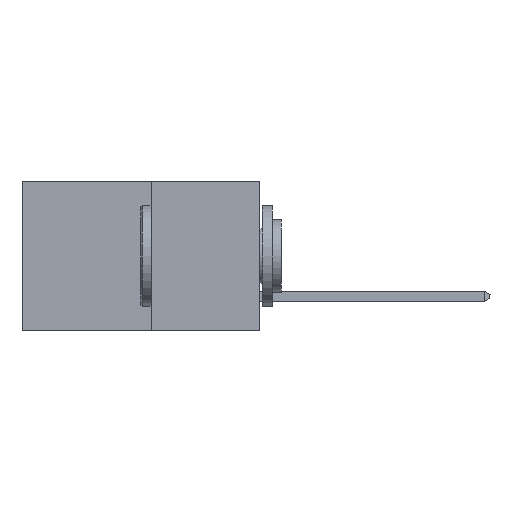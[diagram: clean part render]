
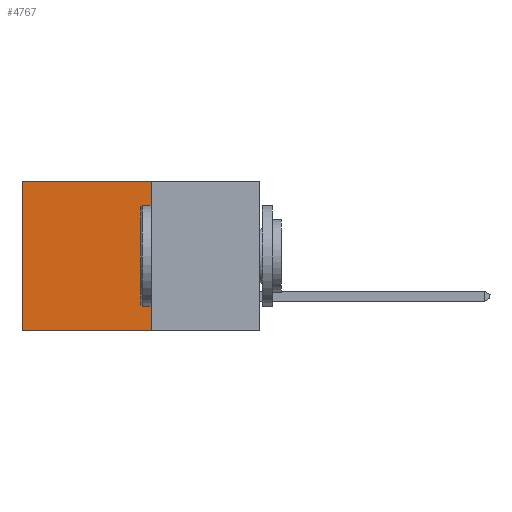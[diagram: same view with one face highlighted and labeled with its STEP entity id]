
A CAD part, left-side view. The second image highlights one B-rep face of the part: STEP entity #4767.
In plain terms, the highlighted planar face has unit normal (-1, 0, 0).
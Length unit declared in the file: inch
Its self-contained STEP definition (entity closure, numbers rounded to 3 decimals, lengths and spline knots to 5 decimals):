
#166 = CARTESIAN_POINT ( 'NONE',  ( 0.277, 0.27, -0.37 ) ) ;
#188 = CARTESIAN_POINT ( 'NONE',  ( 0.277, 0.27, 0. ) ) ;
#253 = FACE_OUTER_BOUND ( 'NONE', #12273, .T. ) ;
#357 = ORIENTED_EDGE ( 'NONE', *, *, #11550, .T. ) ;
#1456 = VERTEX_POINT ( 'NONE', #166 ) ;
#1568 = VERTEX_POINT ( 'NONE', #2262 ) ;
#2262 = CARTESIAN_POINT ( 'NONE',  ( 0.277, 0.59, -0.37 ) ) ;
#2397 = CARTESIAN_POINT ( 'NONE',  ( 0.277, 0.27, 0. ) ) ;
#2802 = DIRECTION ( 'NONE',  ( 0., 0., -1. ) ) ;
#2937 = CARTESIAN_POINT ( 'NONE',  ( 0.277, 0.27, -0.37 ) ) ;
#4393 = CARTESIAN_POINT ( 'NONE',  ( 0.277, 0.59, -0.37 ) ) ;
#4767 = ADVANCED_FACE ( 'NONE', ( #253 ), #9715, .F. ) ;
#5192 = EDGE_CURVE ( 'NONE', #11693, #1456, #8290, .T. ) ;
#5298 = AXIS2_PLACEMENT_3D ( 'NONE', #9206, #9105, #9101 ) ;
#5322 = CARTESIAN_POINT ( 'NONE',  ( 0.277, 0.27, -0.37 ) ) ;
#5669 = VECTOR ( 'NONE', #2802, 39.37008 ) ;
#5687 = LINE ( 'NONE', #5322, #10612 ) ;
#6065 = LINE ( 'NONE', #188, #10959 ) ;
#6095 = DIRECTION ( 'NONE',  ( 0., 1., 0. ) ) ;
#6388 = VERTEX_POINT ( 'NONE', #8043 ) ;
#7138 = VECTOR ( 'NONE', #8345, 39.37008 ) ;
#7608 = EDGE_CURVE ( 'NONE', #1456, #1568, #5687, .T. ) ;
#8043 = CARTESIAN_POINT ( 'NONE',  ( 0.277, 0.59, 0. ) ) ;
#8290 = LINE ( 'NONE', #2937, #5669 ) ;
#8345 = DIRECTION ( 'NONE',  ( 0., 0., -1. ) ) ;
#8649 = ORIENTED_EDGE ( 'NONE', *, *, #12426, .T. ) ;
#9101 = DIRECTION ( 'NONE',  ( 0., 0., -1. ) ) ;
#9105 = DIRECTION ( 'NONE',  ( 1., 0., 0. ) ) ;
#9206 = CARTESIAN_POINT ( 'NONE',  ( 0.277, 0.27, -0.37 ) ) ;
#9715 = PLANE ( 'NONE',  #5298 ) ;
#10213 = ORIENTED_EDGE ( 'NONE', *, *, #5192, .F. ) ;
#10612 = VECTOR ( 'NONE', #12077, 39.37008 ) ;
#10959 = VECTOR ( 'NONE', #6095, 39.37008 ) ;
#11550 = EDGE_CURVE ( 'NONE', #11693, #6388, #6065, .T. ) ;
#11693 = VERTEX_POINT ( 'NONE', #2397 ) ;
#12077 = DIRECTION ( 'NONE',  ( 0., 1., 0. ) ) ;
#12221 = LINE ( 'NONE', #4393, #7138 ) ;
#12223 = ORIENTED_EDGE ( 'NONE', *, *, #7608, .F. ) ;
#12273 = EDGE_LOOP ( 'NONE', ( #8649, #12223, #10213, #357 ) ) ;
#12426 = EDGE_CURVE ( 'NONE', #6388, #1568, #12221, .T. ) ;
